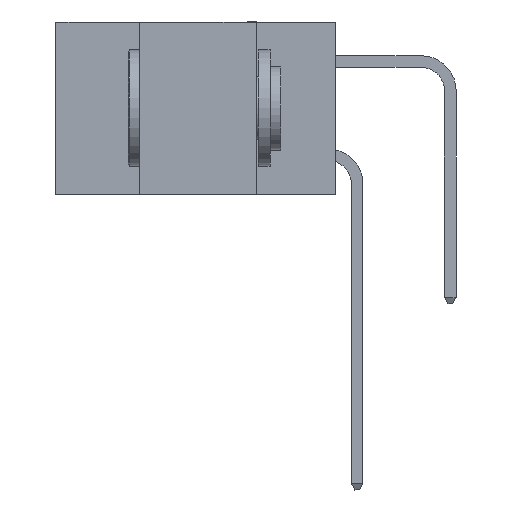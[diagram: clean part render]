
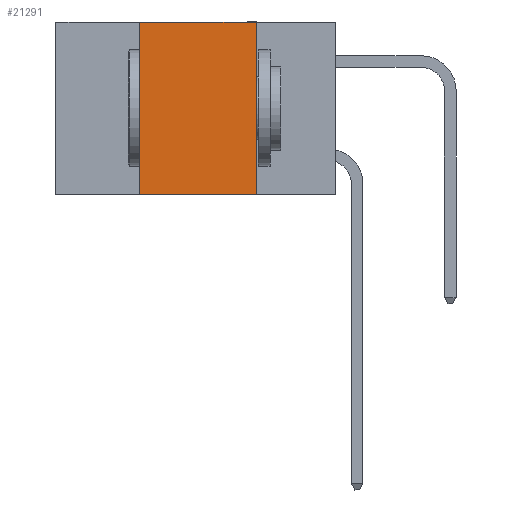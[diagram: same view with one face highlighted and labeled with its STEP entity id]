
A CAD part, left-side view. The second image highlights one B-rep face of the part: STEP entity #21291.
In plain terms, the highlighted planar face has unit normal (-1, 0, 0).
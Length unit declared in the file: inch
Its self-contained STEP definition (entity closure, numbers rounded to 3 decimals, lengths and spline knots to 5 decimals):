
#667 = CARTESIAN_POINT ( 'NONE',  ( 0., 0.42, -0.37 ) ) ;
#2141 = DIRECTION ( 'NONE',  ( 0., -1., 0. ) ) ;
#2480 = CARTESIAN_POINT ( 'NONE',  ( 0., 0.17, 0. ) ) ;
#3135 = CARTESIAN_POINT ( 'NONE',  ( 0., 0.42, 0. ) ) ;
#5151 = CARTESIAN_POINT ( 'NONE',  ( 0., 0.17, -0.37 ) ) ;
#5309 = LINE ( 'NONE', #26497, #18747 ) ;
#5433 = EDGE_CURVE ( 'NONE', #19097, #21630, #5309, .T. ) ;
#6264 = CARTESIAN_POINT ( 'NONE',  ( 0., 0.17, 0. ) ) ;
#6421 = VERTEX_POINT ( 'NONE', #5151 ) ;
#8963 = DIRECTION ( 'NONE',  ( 0., -1., 0. ) ) ;
#9444 = DIRECTION ( 'NONE',  ( 0., 0., 1. ) ) ;
#9952 = ORIENTED_EDGE ( 'NONE', *, *, #18959, .T. ) ;
#10640 = AXIS2_PLACEMENT_3D ( 'NONE', #15253, #17715, #28739 ) ;
#11190 = FACE_OUTER_BOUND ( 'NONE', #14218, .T. ) ;
#14218 = EDGE_LOOP ( 'NONE', ( #32676, #14225, #15493, #9952 ) ) ;
#14225 = ORIENTED_EDGE ( 'NONE', *, *, #5433, .F. ) ;
#15253 = CARTESIAN_POINT ( 'NONE',  ( 0., 0.6, 0. ) ) ;
#15493 = ORIENTED_EDGE ( 'NONE', *, *, #17382, .F. ) ;
#15697 = LINE ( 'NONE', #2480, #18635 ) ;
#17382 = EDGE_CURVE ( 'NONE', #18771, #19097, #20414, .T. ) ;
#17715 = DIRECTION ( 'NONE',  ( 1., 0., 0. ) ) ;
#17955 = PLANE ( 'NONE',  #10640 ) ;
#18132 = CARTESIAN_POINT ( 'NONE',  ( 0., 0.42, 0. ) ) ;
#18217 = LINE ( 'NONE', #20249, #30358 ) ;
#18635 = VECTOR ( 'NONE', #21233, 39.37008 ) ;
#18747 = VECTOR ( 'NONE', #2141, 39.37008 ) ;
#18771 = VERTEX_POINT ( 'NONE', #667 ) ;
#18959 = EDGE_CURVE ( 'NONE', #18771, #6421, #18217, .T. ) ;
#19097 = VERTEX_POINT ( 'NONE', #18132 ) ;
#20249 = CARTESIAN_POINT ( 'NONE',  ( 0., 0.6, -0.37 ) ) ;
#20414 = LINE ( 'NONE', #3135, #31774 ) ;
#21233 = DIRECTION ( 'NONE',  ( 0., 0., -1. ) ) ;
#21291 = ADVANCED_FACE ( 'NONE', ( #11190 ), #17955, .F. ) ;
#21630 = VERTEX_POINT ( 'NONE', #6264 ) ;
#26497 = CARTESIAN_POINT ( 'NONE',  ( 0., 0.6, 0. ) ) ;
#28739 = DIRECTION ( 'NONE',  ( 0., 0., -1. ) ) ;
#30358 = VECTOR ( 'NONE', #8963, 39.37008 ) ;
#31274 = EDGE_CURVE ( 'NONE', #21630, #6421, #15697, .T. ) ;
#31774 = VECTOR ( 'NONE', #9444, 39.37008 ) ;
#32676 = ORIENTED_EDGE ( 'NONE', *, *, #31274, .F. ) ;
